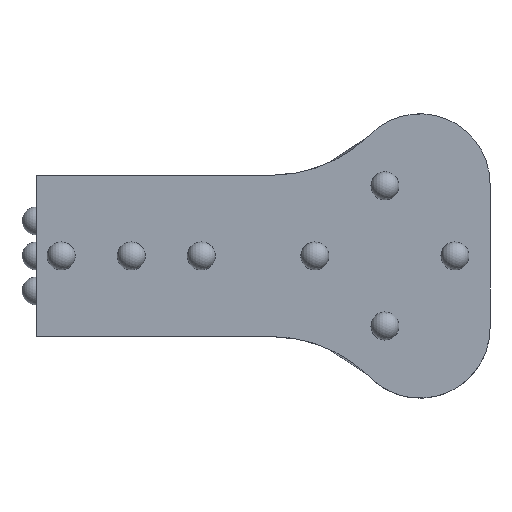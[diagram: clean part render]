
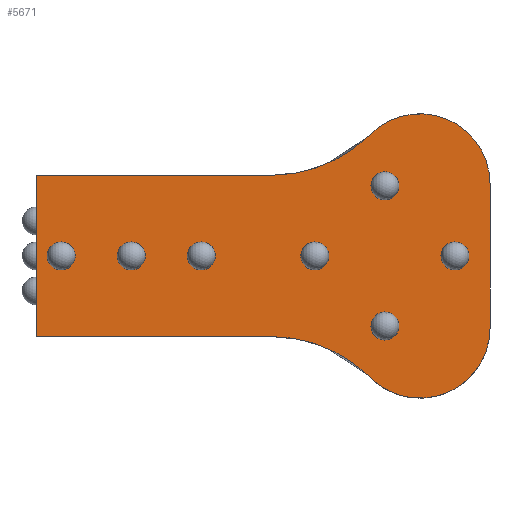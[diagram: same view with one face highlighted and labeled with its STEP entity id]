
A CAD part, left-side view. The second image highlights one B-rep face of the part: STEP entity #5671.
In plain terms, the highlighted planar face has unit normal (-1, 0, 0).
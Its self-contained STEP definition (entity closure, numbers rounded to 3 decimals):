
#5 = CARTESIAN_POINT ( 'NONE',  ( -211.361, -48.733, 36.057 ) ) ;
#68 = ORIENTED_EDGE ( 'NONE', *, *, #5224, .F. ) ;
#286 = VERTEX_POINT ( 'NONE', #6063 ) ;
#291 = CARTESIAN_POINT ( 'NONE',  ( -211.361, -15.145, 458.444 ) ) ;
#338 = CARTESIAN_POINT ( 'NONE',  ( -211.361, -62.943, -5.453 ) ) ;
#354 = CARTESIAN_POINT ( 'NONE',  ( -211.361, -62.943, 14.547 ) ) ;
#370 = DIRECTION ( 'NONE',  ( 0., 1., 0. ) ) ;
#448 = CARTESIAN_POINT ( 'NONE',  ( -211.361, -62.873, -12.817 ) ) ;
#501 = EDGE_CURVE ( 'NONE', #2704, #2704, #4208, .T. ) ;
#505 = DIRECTION ( 'NONE',  ( 0., 0., -1. ) ) ;
#767 = VECTOR ( 'NONE', #4064, 1000. ) ;
#800 = LINE ( 'NONE', #5022, #767 ) ;
#855 = CARTESIAN_POINT ( 'NONE',  ( -211.361, -16.733, 4.547 ) ) ;
#884 = FACE_BOUND ( 'NONE', #5179, .T. ) ;
#889 = AXIS2_PLACEMENT_3D ( 'NONE', #6123, #3798, #944 ) ;
#893 = CARTESIAN_POINT ( 'NONE',  ( -211.361, -79.943, 14.84 ) ) ;
#944 = DIRECTION ( 'NONE',  ( 0., 0., -1. ) ) ;
#959 = FACE_BOUND ( 'NONE', #5331, .T. ) ;
#1000 = AXIS2_PLACEMENT_3D ( 'NONE', #4123, #1266, #4600 ) ;
#1066 = DIRECTION ( 'NONE',  ( -1., 0., 0. ) ) ;
#1123 = VECTOR ( 'NONE', #2162, 1000. ) ;
#1138 = CIRCLE ( 'NONE', #3285, 10. ) ;
#1206 = AXIS2_PLACEMENT_3D ( 'NONE', #2893, #6176, #3355 ) ;
#1266 = DIRECTION ( 'NONE',  ( -1., 0., 0. ) ) ;
#1269 = EDGE_CURVE ( 'NONE', #5741, #5741, #3745, .T. ) ;
#1398 = CARTESIAN_POINT ( 'NONE',  ( -211.361, -64.943, 14.547 ) ) ;
#1407 = DIRECTION ( 'NONE',  ( 0., 0., 1. ) ) ;
#1490 = CARTESIAN_POINT ( 'NONE',  ( -211.361, -38.733, 4.547 ) ) ;
#1524 = EDGE_LOOP ( 'NONE', ( #3299 ) ) ;
#1559 = CARTESIAN_POINT ( 'NONE',  ( -211.361, 231.715, 16.057 ) ) ;
#1606 = VERTEX_POINT ( 'NONE', #2682 ) ;
#1613 = VERTEX_POINT ( 'NONE', #4103 ) ;
#1668 = CARTESIAN_POINT ( 'NONE',  ( -211.361, 231.715, -6.962 ) ) ;
#1698 = DIRECTION ( 'NONE',  ( 0., 1., 0. ) ) ;
#1700 = DIRECTION ( 'NONE',  ( -1., 0., 0. ) ) ;
#1765 = DIRECTION ( 'NONE',  ( -1., 0., 0. ) ) ;
#1785 = CARTESIAN_POINT ( 'NONE',  ( -211.361, -64.943, -5.453 ) ) ;
#1817 = CIRCLE ( 'NONE', #4033, 20. ) ;
#1883 = DIRECTION ( 'NONE',  ( 0., 1., 0. ) ) ;
#1914 = EDGE_CURVE ( 'NONE', #286, #286, #3228, .T. ) ;
#1958 = VECTOR ( 'NONE', #1407, 1000. ) ;
#1976 = LINE ( 'NONE', #291, #1958 ) ;
#1980 = DIRECTION ( 'NONE',  ( 0., 1., 0. ) ) ;
#2119 = EDGE_CURVE ( 'NONE', #2707, #2707, #3079, .T. ) ;
#2150 = VECTOR ( 'NONE', #4021, 1000. ) ;
#2162 = DIRECTION ( 'NONE',  ( 0., 1., 0. ) ) ;
#2258 = AXIS2_PLACEMENT_3D ( 'NONE', #1398, #4732, #1883 ) ;
#2290 = LINE ( 'NONE', #1559, #2150 ) ;
#2302 = AXIS2_PLACEMENT_3D ( 'NONE', #6077, #3257, #370 ) ;
#2350 = CARTESIAN_POINT ( 'NONE',  ( -211.361, -62.873, 21.912 ) ) ;
#2435 = CARTESIAN_POINT ( 'NONE',  ( -211.361, -54.943, 4.547 ) ) ;
#2443 = EDGE_CURVE ( 'NONE', #3435, #3435, #2749, .T. ) ;
#2483 = AXIS2_PLACEMENT_3D ( 'NONE', #1490, #4825, #1980 ) ;
#2557 = EDGE_CURVE ( 'NONE', #5084, #5084, #2590, .T. ) ;
#2590 = CIRCLE ( 'NONE', #4464, 2. ) ;
#2682 = CARTESIAN_POINT ( 'NONE',  ( -211.361, -79.943, -5.745 ) ) ;
#2697 = CARTESIAN_POINT ( 'NONE',  ( -211.361, -28.733, 4.547 ) ) ;
#2704 = VERTEX_POINT ( 'NONE', #338 ) ;
#2707 = VERTEX_POINT ( 'NONE', #3239 ) ;
#2749 = CIRCLE ( 'NONE', #2258, 2. ) ;
#2854 = PLANE ( 'NONE',  #889 ) ;
#2881 = EDGE_CURVE ( 'NONE', #1613, #5557, #2290, .T. ) ;
#2893 = CARTESIAN_POINT ( 'NONE',  ( -211.361, -48.733, -26.962 ) ) ;
#2913 = DIRECTION ( 'NONE',  ( 0., 1., 0. ) ) ;
#3072 = LINE ( 'NONE', #1668, #1123 ) ;
#3079 = CIRCLE ( 'NONE', #5858, 2. ) ;
#3080 = EDGE_CURVE ( 'NONE', #5637, #5557, #1976, .T. ) ;
#3172 = DIRECTION ( 'NONE',  ( 0., 1., 0. ) ) ;
#3204 = EDGE_CURVE ( 'NONE', #1613, #5630, #1817, .T. ) ;
#3228 = CIRCLE ( 'NONE', #3945, 2. ) ;
#3239 = CARTESIAN_POINT ( 'NONE',  ( -211.361, -26.733, 4.547 ) ) ;
#3257 = DIRECTION ( 'NONE',  ( -1., 0., 0. ) ) ;
#3285 = AXIS2_PLACEMENT_3D ( 'NONE', #4546, #1700, #5030 ) ;
#3297 = CARTESIAN_POINT ( 'NONE',  ( -211.361, -15.145, -6.962 ) ) ;
#3299 = ORIENTED_EDGE ( 'NONE', *, *, #2443, .F. ) ;
#3325 = ORIENTED_EDGE ( 'NONE', *, *, #2119, .F. ) ;
#3355 = DIRECTION ( 'NONE',  ( 0., 0., -1. ) ) ;
#3369 = DIRECTION ( 'NONE',  ( -1., 0., 0. ) ) ;
#3404 = EDGE_LOOP ( 'NONE', ( #5636 ) ) ;
#3435 = VERTEX_POINT ( 'NONE', #354 ) ;
#3566 = EDGE_LOOP ( 'NONE', ( #4492 ) ) ;
#3570 = FACE_BOUND ( 'NONE', #3404, .T. ) ;
#3716 = CARTESIAN_POINT ( 'NONE',  ( -211.361, -52.943, 4.547 ) ) ;
#3745 = CIRCLE ( 'NONE', #2483, 2. ) ;
#3759 = CARTESIAN_POINT ( 'NONE',  ( -211.361, -15.145, 16.057 ) ) ;
#3795 = FACE_BOUND ( 'NONE', #1524, .T. ) ;
#3798 = DIRECTION ( 'NONE',  ( 1., 0., 0. ) ) ;
#3824 = EDGE_CURVE ( 'NONE', #4516, #5630, #1138, .T. ) ;
#3923 = CARTESIAN_POINT ( 'NONE',  ( -211.361, -74.943, 4.547 ) ) ;
#3945 = AXIS2_PLACEMENT_3D ( 'NONE', #3923, #1066, #4388 ) ;
#4021 = DIRECTION ( 'NONE',  ( 0., 1., 0. ) ) ;
#4033 = AXIS2_PLACEMENT_3D ( 'NONE', #5, #3369, #505 ) ;
#4064 = DIRECTION ( 'NONE',  ( 0., 0., -1. ) ) ;
#4103 = CARTESIAN_POINT ( 'NONE',  ( -211.361, -48.733, 16.057 ) ) ;
#4123 = CARTESIAN_POINT ( 'NONE',  ( -211.361, -69.943, -5.745 ) ) ;
#4148 = EDGE_CURVE ( 'NONE', #4516, #1606, #800, .T. ) ;
#4208 = CIRCLE ( 'NONE', #4629, 2. ) ;
#4388 = DIRECTION ( 'NONE',  ( 0., 1., 0. ) ) ;
#4464 = AXIS2_PLACEMENT_3D ( 'NONE', #2435, #5753, #2913 ) ;
#4470 = VERTEX_POINT ( 'NONE', #855 ) ;
#4492 = ORIENTED_EDGE ( 'NONE', *, *, #501, .F. ) ;
#4510 = VERTEX_POINT ( 'NONE', #4699 ) ;
#4516 = VERTEX_POINT ( 'NONE', #893 ) ;
#4520 = ORIENTED_EDGE ( 'NONE', *, *, #3080, .F. ) ;
#4546 = CARTESIAN_POINT ( 'NONE',  ( -211.361, -69.943, 14.84 ) ) ;
#4576 = ORIENTED_EDGE ( 'NONE', *, *, #6043, .F. ) ;
#4600 = DIRECTION ( 'NONE',  ( 0., 0., -1. ) ) ;
#4615 = FACE_BOUND ( 'NONE', #5719, .T. ) ;
#4621 = FACE_OUTER_BOUND ( 'NONE', #5575, .T. ) ;
#4629 = AXIS2_PLACEMENT_3D ( 'NONE', #1785, #1765, #1698 ) ;
#4656 = ORIENTED_EDGE ( 'NONE', *, *, #5740, .F. ) ;
#4699 = CARTESIAN_POINT ( 'NONE',  ( -211.361, -48.733, -6.962 ) ) ;
#4732 = DIRECTION ( 'NONE',  ( -1., 0., 0. ) ) ;
#4825 = DIRECTION ( 'NONE',  ( -1., 0., 0. ) ) ;
#5021 = ORIENTED_EDGE ( 'NONE', *, *, #5109, .T. ) ;
#5022 = CARTESIAN_POINT ( 'NONE',  ( -211.361, -79.943, -21.728 ) ) ;
#5030 = DIRECTION ( 'NONE',  ( 0., 0., -1. ) ) ;
#5058 = ORIENTED_EDGE ( 'NONE', *, *, #4148, .F. ) ;
#5084 = VERTEX_POINT ( 'NONE', #3716 ) ;
#5109 = EDGE_CURVE ( 'NONE', #5688, #1606, #5594, .T. ) ;
#5128 = ORIENTED_EDGE ( 'NONE', *, *, #3824, .T. ) ;
#5165 = ORIENTED_EDGE ( 'NONE', *, *, #3204, .F. ) ;
#5179 = EDGE_LOOP ( 'NONE', ( #3325 ) ) ;
#5209 = FACE_BOUND ( 'NONE', #3566, .T. ) ;
#5224 = EDGE_CURVE ( 'NONE', #4470, #4470, #6015, .T. ) ;
#5331 = EDGE_LOOP ( 'NONE', ( #5769 ) ) ;
#5557 = VERTEX_POINT ( 'NONE', #3759 ) ;
#5575 = EDGE_LOOP ( 'NONE', ( #4520, #4576, #4656, #5021, #5058, #5128, #5165, #5581 ) ) ;
#5581 = ORIENTED_EDGE ( 'NONE', *, *, #2881, .T. ) ;
#5594 = CIRCLE ( 'NONE', #1000, 10. ) ;
#5618 = CARTESIAN_POINT ( 'NONE',  ( -211.361, -36.733, 4.547 ) ) ;
#5630 = VERTEX_POINT ( 'NONE', #2350 ) ;
#5636 = ORIENTED_EDGE ( 'NONE', *, *, #1914, .F. ) ;
#5637 = VERTEX_POINT ( 'NONE', #3297 ) ;
#5671 = ADVANCED_FACE ( 'NONE', ( #884, #5209, #3795, #4621, #959, #3570, #4615, #5940 ), #2854, .F. ) ;
#5686 = EDGE_LOOP ( 'NONE', ( #68 ) ) ;
#5688 = VERTEX_POINT ( 'NONE', #448 ) ;
#5694 = ORIENTED_EDGE ( 'NONE', *, *, #1269, .F. ) ;
#5719 = EDGE_LOOP ( 'NONE', ( #5694 ) ) ;
#5740 = EDGE_CURVE ( 'NONE', #5688, #4510, #6160, .T. ) ;
#5741 = VERTEX_POINT ( 'NONE', #5618 ) ;
#5753 = DIRECTION ( 'NONE',  ( -1., 0., 0. ) ) ;
#5769 = ORIENTED_EDGE ( 'NONE', *, *, #2557, .F. ) ;
#5858 = AXIS2_PLACEMENT_3D ( 'NONE', #2697, #5998, #3172 ) ;
#5940 = FACE_BOUND ( 'NONE', #5686, .T. ) ;
#5998 = DIRECTION ( 'NONE',  ( -1., 0., 0. ) ) ;
#6015 = CIRCLE ( 'NONE', #2302, 2. ) ;
#6043 = EDGE_CURVE ( 'NONE', #4510, #5637, #3072, .T. ) ;
#6063 = CARTESIAN_POINT ( 'NONE',  ( -211.361, -72.943, 4.547 ) ) ;
#6077 = CARTESIAN_POINT ( 'NONE',  ( -211.361, -18.733, 4.547 ) ) ;
#6123 = CARTESIAN_POINT ( 'NONE',  ( -211.361, 140.231, 458.444 ) ) ;
#6160 = CIRCLE ( 'NONE', #1206, 20. ) ;
#6176 = DIRECTION ( 'NONE',  ( -1., 0., 0. ) ) ;
